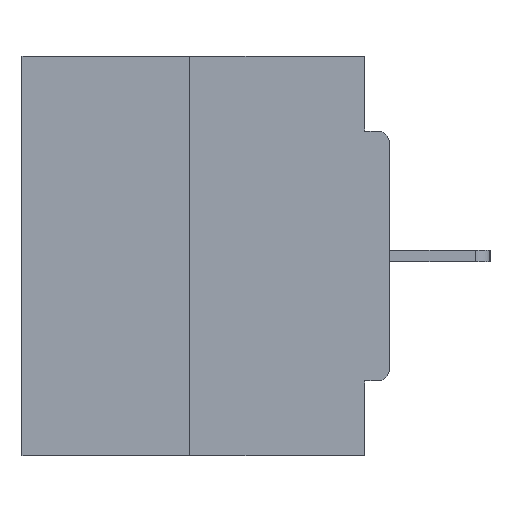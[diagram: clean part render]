
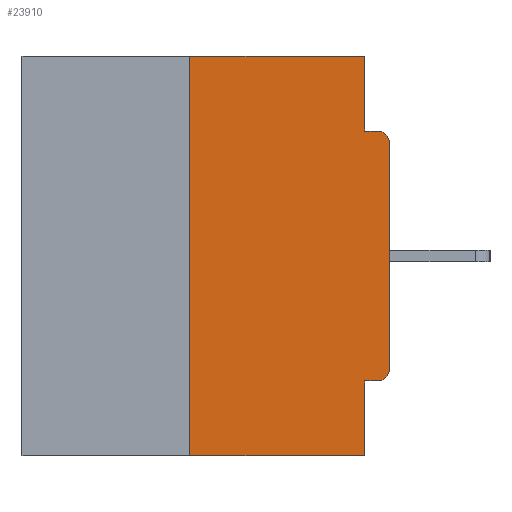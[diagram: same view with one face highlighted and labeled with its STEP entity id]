
A CAD part, left-side view. The second image highlights one B-rep face of the part: STEP entity #23910.
In plain terms, the highlighted planar face has unit normal (-1, 0, 0).
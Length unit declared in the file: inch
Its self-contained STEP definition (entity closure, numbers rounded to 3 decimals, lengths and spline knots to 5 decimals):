
#92 = ORIENTED_EDGE ( 'NONE', *, *, #2168, .F. ) ;
#836 = EDGE_CURVE ( 'NONE', #18707, #30877, #16875, .T. ) ;
#1106 = DIRECTION ( 'NONE',  ( 0., 0., -1. ) ) ;
#1145 = VECTOR ( 'NONE', #24323, 39.37008 ) ;
#1596 = CARTESIAN_POINT ( 'NONE',  ( 0., 0.25, 0. ) ) ;
#1763 = ORIENTED_EDGE ( 'NONE', *, *, #836, .F. ) ;
#1803 = VERTEX_POINT ( 'NONE', #9671 ) ;
#1814 = EDGE_CURVE ( 'NONE', #19400, #27838, #6482, .T. ) ;
#2114 = ORIENTED_EDGE ( 'NONE', *, *, #5987, .T. ) ;
#2168 = EDGE_CURVE ( 'NONE', #30274, #19400, #39071, .T. ) ;
#2219 = AXIS2_PLACEMENT_3D ( 'NONE', #21029, #32833, #36039 ) ;
#2274 = CARTESIAN_POINT ( 'NONE',  ( 0., 0.25, 0. ) ) ;
#2933 = EDGE_CURVE ( 'NONE', #12112, #15661, #22710, .T. ) ;
#2934 = CARTESIAN_POINT ( 'NONE',  ( 0., 0.015, -0.1085 ) ) ;
#4462 = LINE ( 'NONE', #8043, #25614 ) ;
#5298 = CARTESIAN_POINT ( 'NONE',  ( 0., 0.015, -0.0935 ) ) ;
#5585 = CARTESIAN_POINT ( 'NONE',  ( 0., 0.031, 0. ) ) ;
#5987 = EDGE_CURVE ( 'NONE', #1803, #7895, #23652, .T. ) ;
#6097 = LINE ( 'NONE', #30077, #35460 ) ;
#6482 = LINE ( 'NONE', #24655, #19037 ) ;
#6668 = DIRECTION ( 'NONE',  ( -1., 0., 0. ) ) ;
#6948 = EDGE_CURVE ( 'NONE', #7895, #30877, #25953, .T. ) ;
#7299 = PLANE ( 'NONE',  #37827 ) ;
#7895 = VERTEX_POINT ( 'NONE', #22146 ) ;
#8043 = CARTESIAN_POINT ( 'NONE',  ( 0., 0.031, 0. ) ) ;
#8785 = ORIENTED_EDGE ( 'NONE', *, *, #18980, .F. ) ;
#9671 = CARTESIAN_POINT ( 'NONE',  ( 0., 0., -0.3915 ) ) ;
#10385 = ORIENTED_EDGE ( 'NONE', *, *, #29242, .T. ) ;
#11219 = CARTESIAN_POINT ( 'NONE',  ( 0., 0.031, -0.5 ) ) ;
#11581 = ORIENTED_EDGE ( 'NONE', *, *, #21618, .T. ) ;
#12051 = ORIENTED_EDGE ( 'NONE', *, *, #2933, .F. ) ;
#12112 = VERTEX_POINT ( 'NONE', #37971 ) ;
#12203 = ORIENTED_EDGE ( 'NONE', *, *, #6948, .T. ) ;
#13474 = DIRECTION ( 'NONE',  ( 1., 0., 0. ) ) ;
#13535 = EDGE_LOOP ( 'NONE', ( #22096, #92, #10385, #33614, #12051, #11581, #2114, #12203, #1763, #8785 ) ) ;
#13854 = VECTOR ( 'NONE', #29235, 39.37008 ) ;
#14038 = EDGE_CURVE ( 'NONE', #15661, #19136, #6097, .T. ) ;
#15221 = VECTOR ( 'NONE', #30211, 39.37008 ) ;
#15661 = VERTEX_POINT ( 'NONE', #31588 ) ;
#16278 = DIRECTION ( 'NONE',  ( 0., -1., 0. ) ) ;
#16546 = DIRECTION ( 'NONE',  ( 0., 1., 0. ) ) ;
#16875 = LINE ( 'NONE', #29034, #13854 ) ;
#18550 = CARTESIAN_POINT ( 'NONE',  ( 0., 0.46, -0.5 ) ) ;
#18707 = VERTEX_POINT ( 'NONE', #33077 ) ;
#18980 = EDGE_CURVE ( 'NONE', #27838, #18707, #4462, .T. ) ;
#19037 = VECTOR ( 'NONE', #16278, 39.37008 ) ;
#19136 = VERTEX_POINT ( 'NONE', #11219 ) ;
#19400 = VERTEX_POINT ( 'NONE', #1596 ) ;
#21029 = CARTESIAN_POINT ( 'NONE',  ( 0., 0.015, -0.3915 ) ) ;
#21618 = EDGE_CURVE ( 'NONE', #12112, #1803, #23247, .T. ) ;
#22069 = VECTOR ( 'NONE', #35876, 39.37008 ) ;
#22096 = ORIENTED_EDGE ( 'NONE', *, *, #1814, .F. ) ;
#22146 = CARTESIAN_POINT ( 'NONE',  ( 0., 0., -0.1085 ) ) ;
#22710 = LINE ( 'NONE', #29098, #32417 ) ;
#23013 = DIRECTION ( 'NONE',  ( 0., 0., -1. ) ) ;
#23247 = CIRCLE ( 'NONE', #2219, 0.015 ) ;
#23652 = LINE ( 'NONE', #39092, #22069 ) ;
#23910 = ADVANCED_FACE ( 'NONE', ( #37705 ), #7299, .F. ) ;
#24323 = DIRECTION ( 'NONE',  ( 0., -1., 0. ) ) ;
#24655 = CARTESIAN_POINT ( 'NONE',  ( 0., 0.46, 0. ) ) ;
#25614 = VECTOR ( 'NONE', #23013, 39.37008 ) ;
#25851 = CARTESIAN_POINT ( 'NONE',  ( 0., 0.46, 0. ) ) ;
#25953 = CIRCLE ( 'NONE', #31074, 0.015 ) ;
#27296 = DIRECTION ( 'NONE',  ( 0., 0., -1. ) ) ;
#27650 = DIRECTION ( 'NONE',  ( 0., 0., -1. ) ) ;
#27838 = VERTEX_POINT ( 'NONE', #5585 ) ;
#29034 = CARTESIAN_POINT ( 'NONE',  ( 0., 0., -0.0935 ) ) ;
#29098 = CARTESIAN_POINT ( 'NONE',  ( 0., 0., -0.4065 ) ) ;
#29235 = DIRECTION ( 'NONE',  ( 0., -1., 0. ) ) ;
#29242 = EDGE_CURVE ( 'NONE', #30274, #19136, #33944, .T. ) ;
#30077 = CARTESIAN_POINT ( 'NONE',  ( 0., 0.031, -0.5 ) ) ;
#30143 = CARTESIAN_POINT ( 'NONE',  ( 0., 0.25, -0.5 ) ) ;
#30211 = DIRECTION ( 'NONE',  ( 0., 0., 1. ) ) ;
#30274 = VERTEX_POINT ( 'NONE', #30143 ) ;
#30877 = VERTEX_POINT ( 'NONE', #5298 ) ;
#31074 = AXIS2_PLACEMENT_3D ( 'NONE', #2934, #6668, #27296 ) ;
#31588 = CARTESIAN_POINT ( 'NONE',  ( 0., 0.031, -0.4065 ) ) ;
#32417 = VECTOR ( 'NONE', #16546, 39.37008 ) ;
#32833 = DIRECTION ( 'NONE',  ( -1., 0., 0. ) ) ;
#33077 = CARTESIAN_POINT ( 'NONE',  ( 0., 0.031, -0.0935 ) ) ;
#33614 = ORIENTED_EDGE ( 'NONE', *, *, #14038, .F. ) ;
#33944 = LINE ( 'NONE', #18550, #1145 ) ;
#35460 = VECTOR ( 'NONE', #27650, 39.37008 ) ;
#35876 = DIRECTION ( 'NONE',  ( 0., 0., 1. ) ) ;
#36039 = DIRECTION ( 'NONE',  ( 0., 0., -1. ) ) ;
#37705 = FACE_OUTER_BOUND ( 'NONE', #13535, .T. ) ;
#37827 = AXIS2_PLACEMENT_3D ( 'NONE', #25851, #13474, #1106 ) ;
#37971 = CARTESIAN_POINT ( 'NONE',  ( 0., 0.015, -0.4065 ) ) ;
#39071 = LINE ( 'NONE', #2274, #15221 ) ;
#39092 = CARTESIAN_POINT ( 'NONE',  ( 0., 0., 0. ) ) ;
